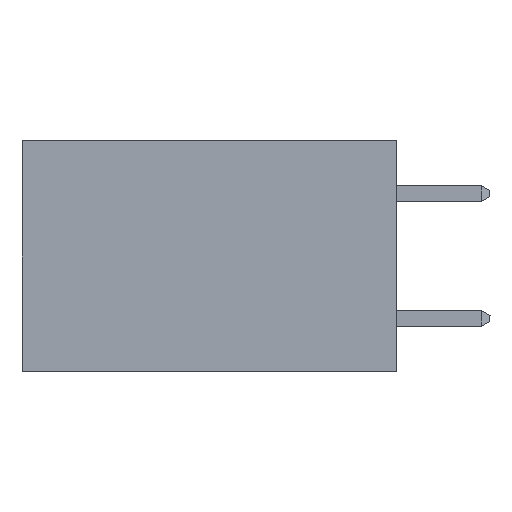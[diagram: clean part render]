
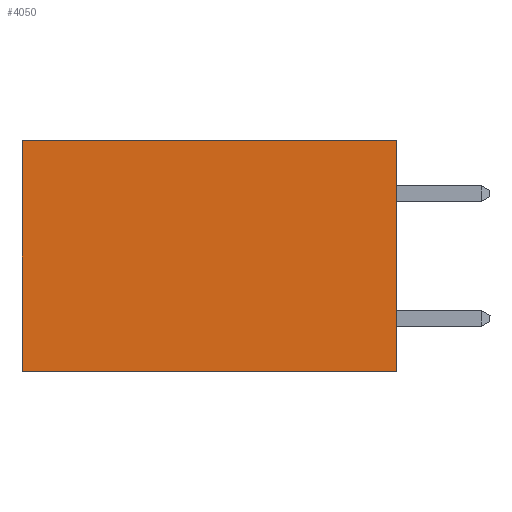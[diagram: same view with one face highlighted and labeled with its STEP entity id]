
A CAD part, left-side view. The second image highlights one B-rep face of the part: STEP entity #4050.
In plain terms, the highlighted planar face has unit normal (-1, 0, 0).
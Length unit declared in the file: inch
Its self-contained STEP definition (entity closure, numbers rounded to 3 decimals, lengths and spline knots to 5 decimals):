
#784 = LINE ( 'NONE', #2906, #5824 ) ;
#1763 = VERTEX_POINT ( 'NONE', #23436 ) ;
#1956 = LINE ( 'NONE', #2087, #11416 ) ;
#2087 = CARTESIAN_POINT ( 'NONE',  ( 0.2615, 0.6, -0.37 ) ) ;
#2452 = LINE ( 'NONE', #15712, #17377 ) ;
#2906 = CARTESIAN_POINT ( 'NONE',  ( 0.2615, 0., -0.37 ) ) ;
#3077 = CARTESIAN_POINT ( 'NONE',  ( 0.2615, 0.6, 0. ) ) ;
#4002 = DIRECTION ( 'NONE',  ( 0., 0., -1. ) ) ;
#4050 = ADVANCED_FACE ( 'NONE', ( #4433 ), #4156, .F. ) ;
#4156 = PLANE ( 'NONE',  #15513 ) ;
#4433 = FACE_OUTER_BOUND ( 'NONE', #6457, .T. ) ;
#4496 = VERTEX_POINT ( 'NONE', #14726 ) ;
#5824 = VECTOR ( 'NONE', #12318, 39.37008 ) ;
#6003 = EDGE_CURVE ( 'NONE', #21552, #17555, #1956, .T. ) ;
#6457 = EDGE_LOOP ( 'NONE', ( #15745, #12850, #23323, #8285 ) ) ;
#7020 = LINE ( 'NONE', #14768, #11449 ) ;
#7940 = DIRECTION ( 'NONE',  ( 1., 0., 0. ) ) ;
#8285 = ORIENTED_EDGE ( 'NONE', *, *, #19258, .T. ) ;
#9654 = CARTESIAN_POINT ( 'NONE',  ( 0.2615, 0.6, -0.37 ) ) ;
#11416 = VECTOR ( 'NONE', #4002, 39.37008 ) ;
#11449 = VECTOR ( 'NONE', #16597, 39.37008 ) ;
#12318 = DIRECTION ( 'NONE',  ( 0., 1., 0. ) ) ;
#12850 = ORIENTED_EDGE ( 'NONE', *, *, #16471, .F. ) ;
#14726 = CARTESIAN_POINT ( 'NONE',  ( 0.2615, 0., -0.37 ) ) ;
#14768 = CARTESIAN_POINT ( 'NONE',  ( 0.2615, 0., -0.37 ) ) ;
#15513 = AXIS2_PLACEMENT_3D ( 'NONE', #19084, #7940, #20954 ) ;
#15712 = CARTESIAN_POINT ( 'NONE',  ( 0.2615, 0., 0. ) ) ;
#15745 = ORIENTED_EDGE ( 'NONE', *, *, #6003, .T. ) ;
#15963 = EDGE_CURVE ( 'NONE', #1763, #4496, #7020, .T. ) ;
#16471 = EDGE_CURVE ( 'NONE', #4496, #17555, #784, .T. ) ;
#16597 = DIRECTION ( 'NONE',  ( 0., 0., -1. ) ) ;
#17377 = VECTOR ( 'NONE', #17568, 39.37008 ) ;
#17555 = VERTEX_POINT ( 'NONE', #9654 ) ;
#17568 = DIRECTION ( 'NONE',  ( 0., 1., 0. ) ) ;
#19084 = CARTESIAN_POINT ( 'NONE',  ( 0.2615, 0., -0.37 ) ) ;
#19258 = EDGE_CURVE ( 'NONE', #1763, #21552, #2452, .T. ) ;
#20954 = DIRECTION ( 'NONE',  ( 0., 0., -1. ) ) ;
#21552 = VERTEX_POINT ( 'NONE', #3077 ) ;
#23323 = ORIENTED_EDGE ( 'NONE', *, *, #15963, .F. ) ;
#23436 = CARTESIAN_POINT ( 'NONE',  ( 0.2615, 0., 0. ) ) ;
